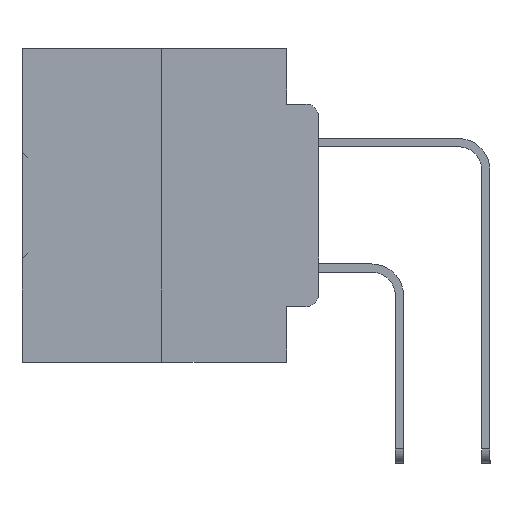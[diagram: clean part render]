
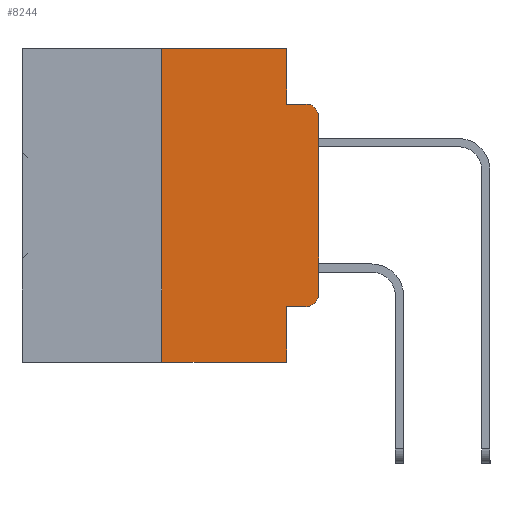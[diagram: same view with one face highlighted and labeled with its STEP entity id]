
A CAD part, left-side view. The second image highlights one B-rep face of the part: STEP entity #8244.
In plain terms, the highlighted planar face has unit normal (-1, 0, 0).
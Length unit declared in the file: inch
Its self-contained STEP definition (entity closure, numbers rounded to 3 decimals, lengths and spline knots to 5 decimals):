
#111 = CARTESIAN_POINT ( 'NONE',  ( 0., 0.473, 0. ) ) ;
#248 = DIRECTION ( 'NONE',  ( 0., 0., -1. ) ) ;
#254 = ORIENTED_EDGE ( 'NONE', *, *, #37542, .T. ) ;
#391 = CARTESIAN_POINT ( 'NONE',  ( 0., 0., -0.1085 ) ) ;
#521 = DIRECTION ( 'NONE',  ( 0., -1., 0. ) ) ;
#688 = ORIENTED_EDGE ( 'NONE', *, *, #25335, .F. ) ;
#798 = ORIENTED_EDGE ( 'NONE', *, *, #7386, .T. ) ;
#1098 = ORIENTED_EDGE ( 'NONE', *, *, #31236, .T. ) ;
#1527 = CARTESIAN_POINT ( 'NONE',  ( 0., 0.051, 0. ) ) ;
#1596 = VERTEX_POINT ( 'NONE', #32023 ) ;
#2786 = DIRECTION ( 'NONE',  ( 0., 0., -1. ) ) ;
#2939 = VERTEX_POINT ( 'NONE', #34556 ) ;
#3509 = VERTEX_POINT ( 'NONE', #10627 ) ;
#4766 = AXIS2_PLACEMENT_3D ( 'NONE', #31207, #13895, #34101 ) ;
#4772 = ORIENTED_EDGE ( 'NONE', *, *, #32961, .F. ) ;
#4989 = EDGE_CURVE ( 'NONE', #5842, #25938, #22145, .T. ) ;
#5067 = LINE ( 'NONE', #34395, #33230 ) ;
#5544 = CARTESIAN_POINT ( 'NONE',  ( 0., 0.051, -0.0885 ) ) ;
#5842 = VERTEX_POINT ( 'NONE', #35722 ) ;
#6222 = LINE ( 'NONE', #5544, #28555 ) ;
#7386 = EDGE_CURVE ( 'NONE', #3509, #24468, #5067, .T. ) ;
#8155 = CARTESIAN_POINT ( 'NONE',  ( 0., 0.02, -0.0885 ) ) ;
#8244 = ADVANCED_FACE ( 'NONE', ( #15558 ), #35091, .F. ) ;
#8549 = DIRECTION ( 'NONE',  ( 0., -1., 0. ) ) ;
#8685 = CARTESIAN_POINT ( 'NONE',  ( 0., 0., -0.3915 ) ) ;
#9623 = VERTEX_POINT ( 'NONE', #391 ) ;
#10627 = CARTESIAN_POINT ( 'NONE',  ( 0., 0.051, -0.4115 ) ) ;
#10733 = LINE ( 'NONE', #14131, #16653 ) ;
#11271 = CIRCLE ( 'NONE', #29882, 0.02 ) ;
#11572 = DIRECTION ( 'NONE',  ( 0., 0., -1. ) ) ;
#12508 = DIRECTION ( 'NONE',  ( 0., -1., 0. ) ) ;
#13895 = DIRECTION ( 'NONE',  ( -1., 0., 0. ) ) ;
#14131 = CARTESIAN_POINT ( 'NONE',  ( 0., 0.25, 0. ) ) ;
#14380 = VECTOR ( 'NONE', #2786, 39.37008 ) ;
#14832 = EDGE_CURVE ( 'NONE', #25938, #29462, #6222, .T. ) ;
#15558 = FACE_OUTER_BOUND ( 'NONE', #26014, .T. ) ;
#15920 = ORIENTED_EDGE ( 'NONE', *, *, #35690, .F. ) ;
#15922 = DIRECTION ( 'NONE',  ( -1., 0., 0. ) ) ;
#16653 = VECTOR ( 'NONE', #37164, 39.37008 ) ;
#17032 = CARTESIAN_POINT ( 'NONE',  ( 0., 0.051, -0.5 ) ) ;
#17484 = VECTOR ( 'NONE', #521, 39.37008 ) ;
#17871 = DIRECTION ( 'NONE',  ( 1., 0., 0. ) ) ;
#19835 = ORIENTED_EDGE ( 'NONE', *, *, #4989, .F. ) ;
#20087 = DIRECTION ( 'NONE',  ( 0., -1., 0. ) ) ;
#20147 = ORIENTED_EDGE ( 'NONE', *, *, #14832, .F. ) ;
#20653 = ORIENTED_EDGE ( 'NONE', *, *, #22677, .T. ) ;
#21465 = ORIENTED_EDGE ( 'NONE', *, *, #30353, .T. ) ;
#22145 = LINE ( 'NONE', #1527, #14380 ) ;
#22677 = EDGE_CURVE ( 'NONE', #9623, #29462, #27031, .T. ) ;
#23408 = CARTESIAN_POINT ( 'NONE',  ( 0., 0.051, -0.0885 ) ) ;
#23781 = VECTOR ( 'NONE', #12508, 39.37008 ) ;
#24254 = CARTESIAN_POINT ( 'NONE',  ( 0., 0.473, -0.5 ) ) ;
#24468 = VERTEX_POINT ( 'NONE', #24646 ) ;
#24646 = CARTESIAN_POINT ( 'NONE',  ( 0., 0.02, -0.4115 ) ) ;
#25026 = VECTOR ( 'NONE', #29417, 39.37008 ) ;
#25050 = AXIS2_PLACEMENT_3D ( 'NONE', #111, #17871, #248 ) ;
#25216 = LINE ( 'NONE', #26771, #17484 ) ;
#25335 = EDGE_CURVE ( 'NONE', #3509, #30156, #30889, .T. ) ;
#25938 = VERTEX_POINT ( 'NONE', #23408 ) ;
#25942 = LINE ( 'NONE', #26552, #25026 ) ;
#26014 = EDGE_LOOP ( 'NONE', ( #21465, #20653, #20147, #19835, #15920, #4772, #254, #688, #798, #1098 ) ) ;
#26552 = CARTESIAN_POINT ( 'NONE',  ( 0., 0., 0. ) ) ;
#26771 = CARTESIAN_POINT ( 'NONE',  ( 0., 0.473, 0. ) ) ;
#27031 = CIRCLE ( 'NONE', #4766, 0.02 ) ;
#28555 = VECTOR ( 'NONE', #8549, 39.37008 ) ;
#29417 = DIRECTION ( 'NONE',  ( 0., 0., 1. ) ) ;
#29462 = VERTEX_POINT ( 'NONE', #8155 ) ;
#29882 = AXIS2_PLACEMENT_3D ( 'NONE', #33214, #15922, #36060 ) ;
#30156 = VERTEX_POINT ( 'NONE', #17032 ) ;
#30353 = EDGE_CURVE ( 'NONE', #32345, #9623, #25942, .T. ) ;
#30889 = LINE ( 'NONE', #31833, #37564 ) ;
#31207 = CARTESIAN_POINT ( 'NONE',  ( 0., 0.02, -0.1085 ) ) ;
#31236 = EDGE_CURVE ( 'NONE', #24468, #32345, #11271, .T. ) ;
#31833 = CARTESIAN_POINT ( 'NONE',  ( 0., 0.051, 0. ) ) ;
#32023 = CARTESIAN_POINT ( 'NONE',  ( 0., 0.25, -0.5 ) ) ;
#32282 = LINE ( 'NONE', #24254, #23781 ) ;
#32345 = VERTEX_POINT ( 'NONE', #8685 ) ;
#32961 = EDGE_CURVE ( 'NONE', #1596, #2939, #10733, .T. ) ;
#33214 = CARTESIAN_POINT ( 'NONE',  ( 0., 0.02, -0.3915 ) ) ;
#33230 = VECTOR ( 'NONE', #20087, 39.37008 ) ;
#34101 = DIRECTION ( 'NONE',  ( 0., 0., -1. ) ) ;
#34395 = CARTESIAN_POINT ( 'NONE',  ( 0., 0.051, -0.4115 ) ) ;
#34556 = CARTESIAN_POINT ( 'NONE',  ( 0., 0.25, 0. ) ) ;
#35091 = PLANE ( 'NONE',  #25050 ) ;
#35690 = EDGE_CURVE ( 'NONE', #2939, #5842, #25216, .T. ) ;
#35722 = CARTESIAN_POINT ( 'NONE',  ( 0., 0.051, 0. ) ) ;
#36060 = DIRECTION ( 'NONE',  ( 0., 0., -1. ) ) ;
#37164 = DIRECTION ( 'NONE',  ( 0., 0., 1. ) ) ;
#37542 = EDGE_CURVE ( 'NONE', #1596, #30156, #32282, .T. ) ;
#37564 = VECTOR ( 'NONE', #11572, 39.37008 ) ;
